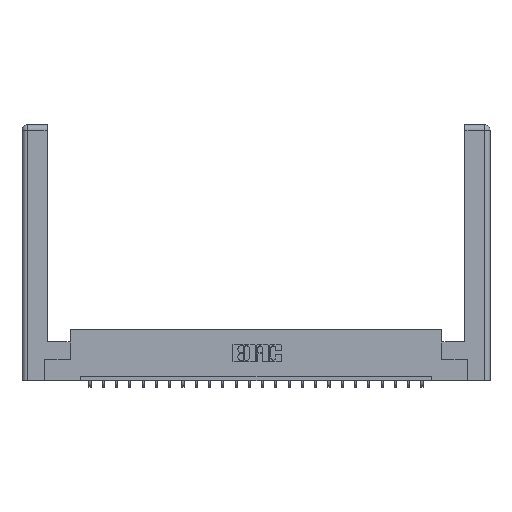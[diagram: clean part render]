
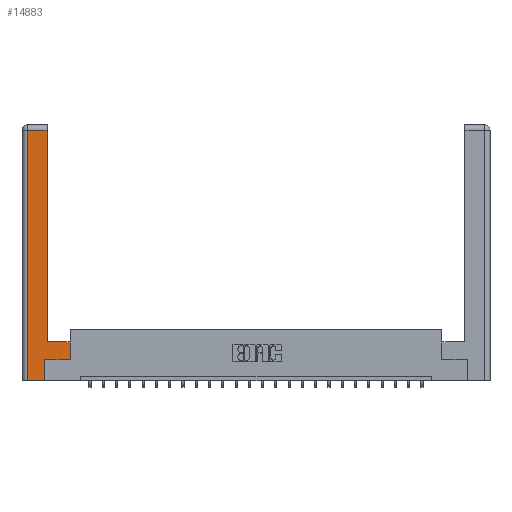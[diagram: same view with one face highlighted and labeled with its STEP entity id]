
A CAD part, top view. The second image highlights one B-rep face of the part: STEP entity #14883.
In plain terms, the highlighted planar face has unit normal (0, 0, 1).
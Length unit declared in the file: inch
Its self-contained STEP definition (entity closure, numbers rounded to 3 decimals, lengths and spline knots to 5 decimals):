
#442 = FACE_OUTER_BOUND ( 'NONE', #22591, .T. ) ;
#767 = CARTESIAN_POINT ( 'NONE',  ( 0., 0., 0. ) ) ;
#966 = CARTESIAN_POINT ( 'NONE',  ( 0.0615, 2.94, 0. ) ) ;
#998 = VECTOR ( 'NONE', #11979, 39.37008 ) ;
#1072 = CARTESIAN_POINT ( 'NONE',  ( 0.565, 0.45, 0. ) ) ;
#1144 = DIRECTION ( 'NONE',  ( 0., 1., 0. ) ) ;
#2228 = DIRECTION ( 'NONE',  ( -1., 0., 0. ) ) ;
#2327 = DIRECTION ( 'NONE',  ( 0., 0., -1. ) ) ;
#2856 = LINE ( 'NONE', #9284, #23871 ) ;
#3118 = CARTESIAN_POINT ( 'NONE',  ( 0.295, 3., 0. ) ) ;
#3136 = CARTESIAN_POINT ( 'NONE',  ( 0.295, 2.94, 0. ) ) ;
#3254 = VERTEX_POINT ( 'NONE', #13625 ) ;
#3863 = VECTOR ( 'NONE', #8527, 39.37008 ) ;
#3870 = VERTEX_POINT ( 'NONE', #12741 ) ;
#4088 = EDGE_CURVE ( 'NONE', #21168, #12572, #23686, .T. ) ;
#4585 = VERTEX_POINT ( 'NONE', #1072 ) ;
#4816 = CARTESIAN_POINT ( 'NONE',  ( 0.565, 0.245, 0. ) ) ;
#5064 = LINE ( 'NONE', #4816, #14964 ) ;
#5249 = ORIENTED_EDGE ( 'NONE', *, *, #6269, .T. ) ;
#5701 = VECTOR ( 'NONE', #17363, 39.37008 ) ;
#6199 = VECTOR ( 'NONE', #15983, 39.37008 ) ;
#6269 = EDGE_CURVE ( 'NONE', #3870, #15135, #14549, .T. ) ;
#6381 = DIRECTION ( 'NONE',  ( 1., 0., 0. ) ) ;
#6438 = CARTESIAN_POINT ( 'NONE',  ( 0.565, 0.45, 0. ) ) ;
#6626 = CARTESIAN_POINT ( 'NONE',  ( 0.265, 0., 0. ) ) ;
#8527 = DIRECTION ( 'NONE',  ( 0., -1., 0. ) ) ;
#8671 = EDGE_CURVE ( 'NONE', #4585, #3870, #9234, .T. ) ;
#9234 = LINE ( 'NONE', #13409, #18555 ) ;
#9284 = CARTESIAN_POINT ( 'NONE',  ( 0.265, 0.245, 0. ) ) ;
#9542 = ORIENTED_EDGE ( 'NONE', *, *, #8671, .T. ) ;
#10110 = CARTESIAN_POINT ( 'NONE',  ( 0.265, 0., 0. ) ) ;
#10342 = CARTESIAN_POINT ( 'NONE',  ( 0.0615, 0., 0. ) ) ;
#11194 = ORIENTED_EDGE ( 'NONE', *, *, #20896, .T. ) ;
#11979 = DIRECTION ( 'NONE',  ( 1., 0., 0. ) ) ;
#12522 = VECTOR ( 'NONE', #1144, 39.37008 ) ;
#12572 = VERTEX_POINT ( 'NONE', #23797 ) ;
#12741 = CARTESIAN_POINT ( 'NONE',  ( 0.295, 0.45, 0. ) ) ;
#13409 = CARTESIAN_POINT ( 'NONE',  ( 0.295, 0.45, 0. ) ) ;
#13625 = CARTESIAN_POINT ( 'NONE',  ( 0.565, 0.245, 0. ) ) ;
#13660 = PLANE ( 'NONE',  #14805 ) ;
#13704 = VERTEX_POINT ( 'NONE', #19381 ) ;
#14549 = LINE ( 'NONE', #3118, #12522 ) ;
#14690 = ORIENTED_EDGE ( 'NONE', *, *, #17565, .T. ) ;
#14805 = AXIS2_PLACEMENT_3D ( 'NONE', #767, #2327, #21073 ) ;
#14883 = ADVANCED_FACE ( 'NONE', ( #442 ), #13660, .F. ) ;
#14964 = VECTOR ( 'NONE', #6381, 39.37008 ) ;
#15135 = VERTEX_POINT ( 'NONE', #3136 ) ;
#15616 = LINE ( 'NONE', #10110, #998 ) ;
#15983 = DIRECTION ( 'NONE',  ( -1., 0., 0. ) ) ;
#16617 = EDGE_CURVE ( 'NONE', #15135, #21168, #18159, .T. ) ;
#17363 = DIRECTION ( 'NONE',  ( 0., 1., 0. ) ) ;
#17565 = EDGE_CURVE ( 'NONE', #3254, #4585, #23748, .T. ) ;
#17629 = EDGE_CURVE ( 'NONE', #12572, #22643, #15616, .T. ) ;
#17784 = ORIENTED_EDGE ( 'NONE', *, *, #4088, .T. ) ;
#18159 = LINE ( 'NONE', #966, #6199 ) ;
#18168 = EDGE_CURVE ( 'NONE', #13704, #3254, #5064, .T. ) ;
#18555 = VECTOR ( 'NONE', #2228, 39.37008 ) ;
#18760 = ORIENTED_EDGE ( 'NONE', *, *, #17629, .T. ) ;
#19381 = CARTESIAN_POINT ( 'NONE',  ( 0.265, 0.245, 0. ) ) ;
#20020 = ORIENTED_EDGE ( 'NONE', *, *, #18168, .T. ) ;
#20896 = EDGE_CURVE ( 'NONE', #22643, #13704, #2856, .T. ) ;
#21073 = DIRECTION ( 'NONE',  ( -1., 0., 0. ) ) ;
#21168 = VERTEX_POINT ( 'NONE', #23756 ) ;
#22392 = DIRECTION ( 'NONE',  ( 0., 1., 0. ) ) ;
#22591 = EDGE_LOOP ( 'NONE', ( #5249, #23219, #17784, #18760, #11194, #20020, #14690, #9542 ) ) ;
#22643 = VERTEX_POINT ( 'NONE', #6626 ) ;
#23219 = ORIENTED_EDGE ( 'NONE', *, *, #16617, .T. ) ;
#23686 = LINE ( 'NONE', #10342, #3863 ) ;
#23748 = LINE ( 'NONE', #6438, #5701 ) ;
#23756 = CARTESIAN_POINT ( 'NONE',  ( 0.0615, 2.94, 0. ) ) ;
#23797 = CARTESIAN_POINT ( 'NONE',  ( 0.0615, 0., 0. ) ) ;
#23871 = VECTOR ( 'NONE', #22392, 39.37008 ) ;
